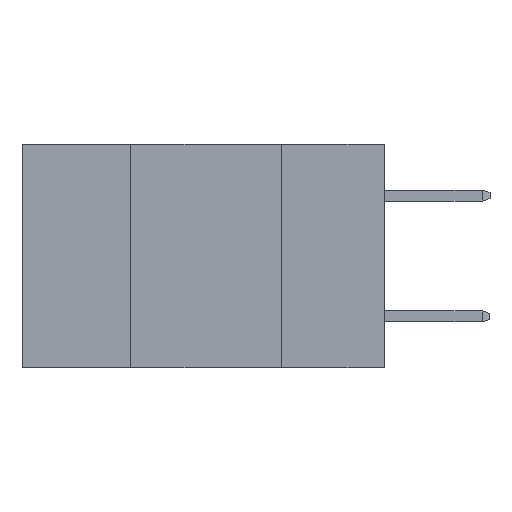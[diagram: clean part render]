
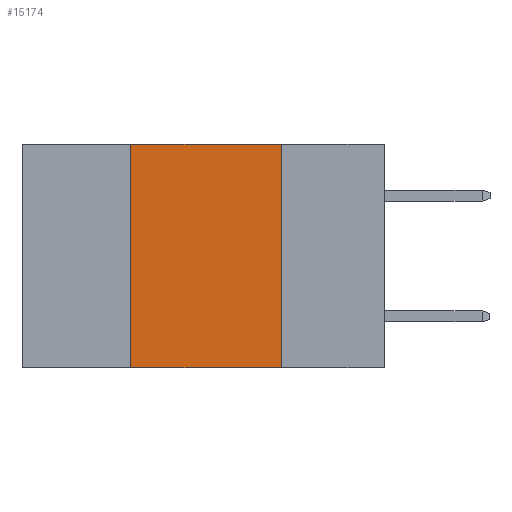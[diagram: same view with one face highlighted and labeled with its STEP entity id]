
A CAD part, left-side view. The second image highlights one B-rep face of the part: STEP entity #15174.
In plain terms, the highlighted planar face has unit normal (-1, 0, 0).
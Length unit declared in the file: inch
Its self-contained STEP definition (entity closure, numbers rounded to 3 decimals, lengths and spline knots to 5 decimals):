
#290 = CARTESIAN_POINT ( 'NONE',  ( 0., 0.6, 0. ) ) ;
#353 = DIRECTION ( 'NONE',  ( 0., -1., 0. ) ) ;
#411 = ORIENTED_EDGE ( 'NONE', *, *, #3791, .F. ) ;
#1602 = EDGE_CURVE ( 'NONE', #6026, #5302, #16986, .T. ) ;
#1623 = VECTOR ( 'NONE', #353, 39.37008 ) ;
#1944 = EDGE_LOOP ( 'NONE', ( #15425, #411, #4116, #5866 ) ) ;
#2042 = VECTOR ( 'NONE', #11930, 39.37008 ) ;
#2652 = AXIS2_PLACEMENT_3D ( 'NONE', #11570, #3265, #12952 ) ;
#3265 = DIRECTION ( 'NONE',  ( 1., 0., 0. ) ) ;
#3791 = EDGE_CURVE ( 'NONE', #5302, #17066, #7769, .T. ) ;
#4116 = ORIENTED_EDGE ( 'NONE', *, *, #1602, .F. ) ;
#5302 = VERTEX_POINT ( 'NONE', #11028 ) ;
#5377 = EDGE_CURVE ( 'NONE', #6026, #9220, #16260, .T. ) ;
#5445 = FACE_OUTER_BOUND ( 'NONE', #1944, .T. ) ;
#5866 = ORIENTED_EDGE ( 'NONE', *, *, #5377, .T. ) ;
#5972 = PLANE ( 'NONE',  #2652 ) ;
#6026 = VERTEX_POINT ( 'NONE', #7164 ) ;
#7164 = CARTESIAN_POINT ( 'NONE',  ( 0., 0.42, -0.37 ) ) ;
#7406 = VECTOR ( 'NONE', #16433, 39.37008 ) ;
#7769 = LINE ( 'NONE', #290, #1623 ) ;
#7950 = CARTESIAN_POINT ( 'NONE',  ( 0., 0.17, 0. ) ) ;
#8597 = VECTOR ( 'NONE', #11195, 39.37008 ) ;
#9220 = VERTEX_POINT ( 'NONE', #11045 ) ;
#10578 = EDGE_CURVE ( 'NONE', #17066, #9220, #17087, .T. ) ;
#11028 = CARTESIAN_POINT ( 'NONE',  ( 0., 0.42, 0. ) ) ;
#11045 = CARTESIAN_POINT ( 'NONE',  ( 0., 0.17, -0.37 ) ) ;
#11195 = DIRECTION ( 'NONE',  ( 0., -1., 0. ) ) ;
#11354 = CARTESIAN_POINT ( 'NONE',  ( 0., 0.17, 0. ) ) ;
#11570 = CARTESIAN_POINT ( 'NONE',  ( 0., 0.6, 0. ) ) ;
#11930 = DIRECTION ( 'NONE',  ( 0., 0., -1. ) ) ;
#12952 = DIRECTION ( 'NONE',  ( 0., 0., -1. ) ) ;
#15174 = ADVANCED_FACE ( 'NONE', ( #5445 ), #5972, .F. ) ;
#15425 = ORIENTED_EDGE ( 'NONE', *, *, #10578, .F. ) ;
#16260 = LINE ( 'NONE', #16592, #8597 ) ;
#16433 = DIRECTION ( 'NONE',  ( 0., 0., 1. ) ) ;
#16592 = CARTESIAN_POINT ( 'NONE',  ( 0., 0.6, -0.37 ) ) ;
#16607 = CARTESIAN_POINT ( 'NONE',  ( 0., 0.42, 0. ) ) ;
#16986 = LINE ( 'NONE', #16607, #7406 ) ;
#17066 = VERTEX_POINT ( 'NONE', #7950 ) ;
#17087 = LINE ( 'NONE', #11354, #2042 ) ;
